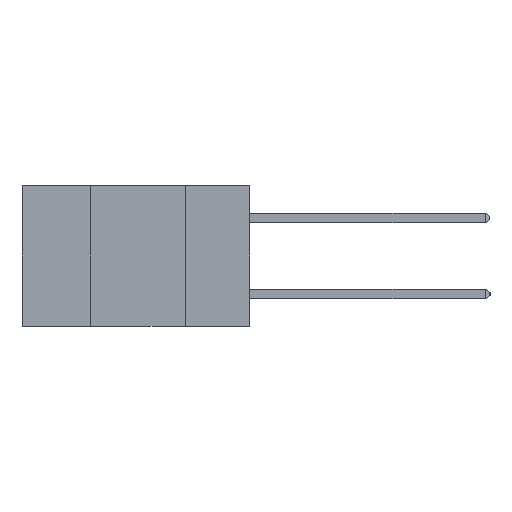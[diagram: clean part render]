
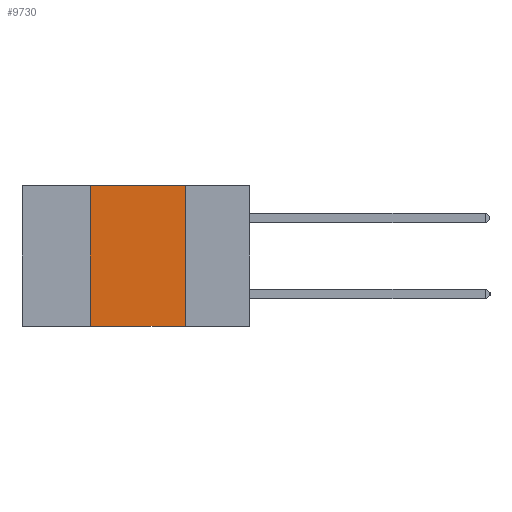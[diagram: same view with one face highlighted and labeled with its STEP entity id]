
A CAD part, left-side view. The second image highlights one B-rep face of the part: STEP entity #9730.
In plain terms, the highlighted planar face has unit normal (-1, 0, 0).
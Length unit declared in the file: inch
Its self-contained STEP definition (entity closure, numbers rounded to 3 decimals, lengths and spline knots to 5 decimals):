
#103 = EDGE_CURVE ( 'NONE', #5767, #11929, #10353, .T. ) ;
#447 = VERTEX_POINT ( 'NONE', #4712 ) ;
#541 = CARTESIAN_POINT ( 'NONE',  ( 0., 0.6, 0. ) ) ;
#1300 = ORIENTED_EDGE ( 'NONE', *, *, #10597, .F. ) ;
#1739 = FACE_OUTER_BOUND ( 'NONE', #11101, .T. ) ;
#1860 = EDGE_CURVE ( 'NONE', #11929, #447, #6072, .T. ) ;
#1995 = ORIENTED_EDGE ( 'NONE', *, *, #103, .F. ) ;
#2318 = DIRECTION ( 'NONE',  ( 0., -1., 0. ) ) ;
#2595 = CARTESIAN_POINT ( 'NONE',  ( 0., 0.42, -0.37 ) ) ;
#2950 = CARTESIAN_POINT ( 'NONE',  ( 0., 0.17, 0. ) ) ;
#3386 = CARTESIAN_POINT ( 'NONE',  ( 0., 0.6, -0.37 ) ) ;
#3473 = CARTESIAN_POINT ( 'NONE',  ( 0., 0.6, 0. ) ) ;
#3732 = ORIENTED_EDGE ( 'NONE', *, *, #1860, .F. ) ;
#3795 = DIRECTION ( 'NONE',  ( 1., 0., 0. ) ) ;
#3872 = DIRECTION ( 'NONE',  ( 0., 0., -1. ) ) ;
#3995 = ORIENTED_EDGE ( 'NONE', *, *, #12463, .T. ) ;
#4287 = DIRECTION ( 'NONE',  ( 0., -1., 0. ) ) ;
#4382 = CARTESIAN_POINT ( 'NONE',  ( 0., 0.42, 0. ) ) ;
#4455 = CARTESIAN_POINT ( 'NONE',  ( 0., 0.17, -0.37 ) ) ;
#4712 = CARTESIAN_POINT ( 'NONE',  ( 0., 0.17, 0. ) ) ;
#5497 = DIRECTION ( 'NONE',  ( 0., 0., 1. ) ) ;
#5767 = VERTEX_POINT ( 'NONE', #2595 ) ;
#6072 = LINE ( 'NONE', #3473, #10510 ) ;
#6585 = VECTOR ( 'NONE', #5497, 39.37008 ) ;
#6977 = VECTOR ( 'NONE', #3872, 39.37008 ) ;
#7831 = DIRECTION ( 'NONE',  ( 0., 0., -1. ) ) ;
#7921 = PLANE ( 'NONE',  #12726 ) ;
#8716 = CARTESIAN_POINT ( 'NONE',  ( 0., 0.42, 0. ) ) ;
#9730 = ADVANCED_FACE ( 'NONE', ( #1739 ), #7921, .F. ) ;
#10042 = LINE ( 'NONE', #3386, #10559 ) ;
#10296 = VERTEX_POINT ( 'NONE', #4455 ) ;
#10353 = LINE ( 'NONE', #4382, #6585 ) ;
#10510 = VECTOR ( 'NONE', #2318, 39.37008 ) ;
#10559 = VECTOR ( 'NONE', #4287, 39.37008 ) ;
#10597 = EDGE_CURVE ( 'NONE', #447, #10296, #13061, .T. ) ;
#11101 = EDGE_LOOP ( 'NONE', ( #1300, #3732, #1995, #3995 ) ) ;
#11929 = VERTEX_POINT ( 'NONE', #8716 ) ;
#12463 = EDGE_CURVE ( 'NONE', #5767, #10296, #10042, .T. ) ;
#12726 = AXIS2_PLACEMENT_3D ( 'NONE', #541, #3795, #7831 ) ;
#13061 = LINE ( 'NONE', #2950, #6977 ) ;
